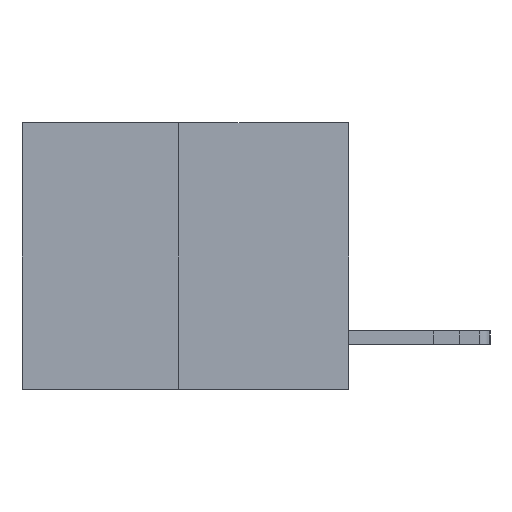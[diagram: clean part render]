
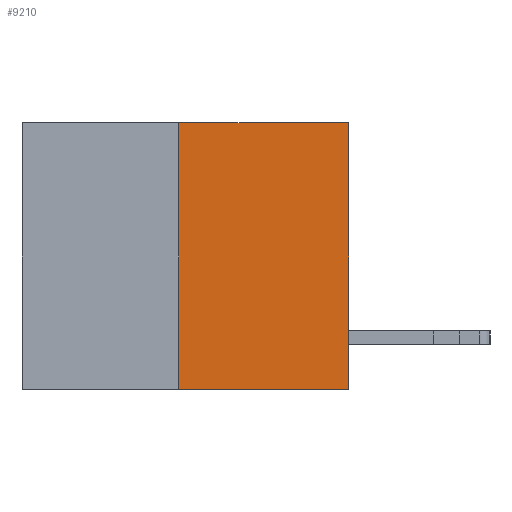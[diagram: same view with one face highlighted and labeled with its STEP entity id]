
A CAD part, left-side view. The second image highlights one B-rep face of the part: STEP entity #9210.
In plain terms, the highlighted planar face has unit normal (-1, 0, 0).
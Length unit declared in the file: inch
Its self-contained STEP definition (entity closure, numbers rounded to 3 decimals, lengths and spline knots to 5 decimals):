
#235 = VERTEX_POINT ( 'NONE', #18334 ) ;
#485 = PLANE ( 'NONE',  #14167 ) ;
#983 = VECTOR ( 'NONE', #2359, 39.37008 ) ;
#1509 = EDGE_CURVE ( 'NONE', #1939, #12032, #9000, .T. ) ;
#1939 = VERTEX_POINT ( 'NONE', #18327 ) ;
#2229 = CARTESIAN_POINT ( 'NONE',  ( 0., 0.6, 0. ) ) ;
#2275 = LINE ( 'NONE', #22118, #2820 ) ;
#2359 = DIRECTION ( 'NONE',  ( 0., 0., 1. ) ) ;
#2820 = VECTOR ( 'NONE', #11802, 39.37008 ) ;
#3719 = ORIENTED_EDGE ( 'NONE', *, *, #1509, .F. ) ;
#3777 = EDGE_LOOP ( 'NONE', ( #10041, #6428, #17152, #3719 ) ) ;
#4070 = CARTESIAN_POINT ( 'NONE',  ( 0., 0., 0. ) ) ;
#6428 = ORIENTED_EDGE ( 'NONE', *, *, #10677, .T. ) ;
#8126 = DIRECTION ( 'NONE',  ( 0., 0., 1. ) ) ;
#9000 = LINE ( 'NONE', #10389, #22377 ) ;
#9210 = ADVANCED_FACE ( 'NONE', ( #15778 ), #485, .F. ) ;
#9233 = CARTESIAN_POINT ( 'NONE',  ( 0., 0., 0. ) ) ;
#9605 = EDGE_CURVE ( 'NONE', #235, #1939, #20968, .T. ) ;
#10041 = ORIENTED_EDGE ( 'NONE', *, *, #9605, .F. ) ;
#10146 = LINE ( 'NONE', #4070, #983 ) ;
#10389 = CARTESIAN_POINT ( 'NONE',  ( 0., 0.6, 0. ) ) ;
#10677 = EDGE_CURVE ( 'NONE', #235, #16303, #2275, .T. ) ;
#11802 = DIRECTION ( 'NONE',  ( 0., -1., 0. ) ) ;
#12032 = VERTEX_POINT ( 'NONE', #9233 ) ;
#12476 = VECTOR ( 'NONE', #8126, 39.37008 ) ;
#12752 = DIRECTION ( 'NONE',  ( 1., 0., 0. ) ) ;
#14167 = AXIS2_PLACEMENT_3D ( 'NONE', #2229, #12752, #17781 ) ;
#14399 = CARTESIAN_POINT ( 'NONE',  ( 0., 0., -0.49 ) ) ;
#15778 = FACE_OUTER_BOUND ( 'NONE', #3777, .T. ) ;
#16303 = VERTEX_POINT ( 'NONE', #14399 ) ;
#17152 = ORIENTED_EDGE ( 'NONE', *, *, #22373, .T. ) ;
#17781 = DIRECTION ( 'NONE',  ( 0., 0., -1. ) ) ;
#18327 = CARTESIAN_POINT ( 'NONE',  ( 0., 0.312, 0. ) ) ;
#18334 = CARTESIAN_POINT ( 'NONE',  ( 0., 0.312, -0.49 ) ) ;
#18895 = DIRECTION ( 'NONE',  ( 0., -1., 0. ) ) ;
#20481 = CARTESIAN_POINT ( 'NONE',  ( 0., 0.312, -0.49 ) ) ;
#20968 = LINE ( 'NONE', #20481, #12476 ) ;
#22118 = CARTESIAN_POINT ( 'NONE',  ( 0., 0.6, -0.49 ) ) ;
#22373 = EDGE_CURVE ( 'NONE', #16303, #12032, #10146, .T. ) ;
#22377 = VECTOR ( 'NONE', #18895, 39.37008 ) ;
